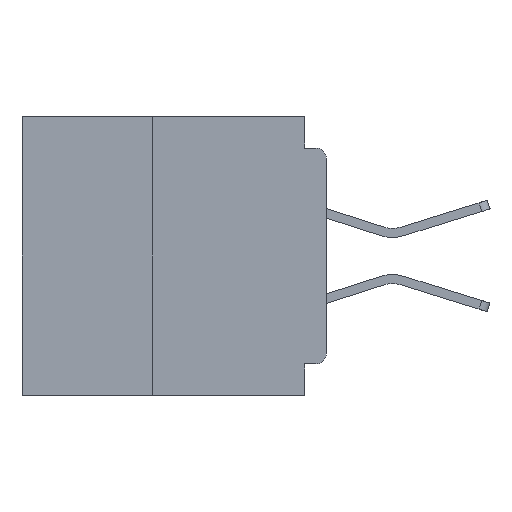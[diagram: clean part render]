
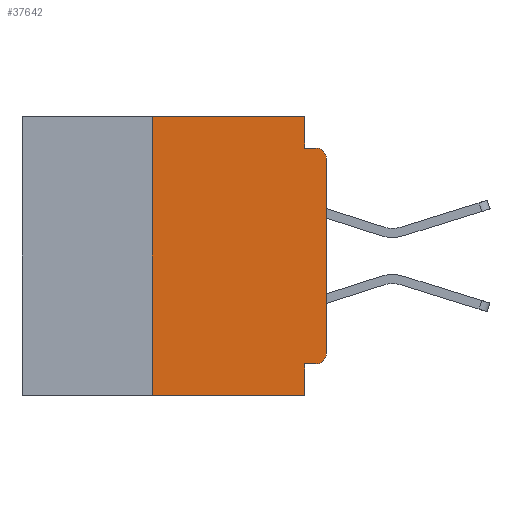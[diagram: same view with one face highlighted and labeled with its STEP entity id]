
A CAD part, left-side view. The second image highlights one B-rep face of the part: STEP entity #37642.
In plain terms, the highlighted planar face has unit normal (-1, 0, 0).
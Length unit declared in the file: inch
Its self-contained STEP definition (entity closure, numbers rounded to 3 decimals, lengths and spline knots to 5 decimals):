
#1137 = CIRCLE ( 'NONE', #14634, 0.015 ) ;
#1537 = VECTOR ( 'NONE', #10099, 39.37008 ) ;
#1831 = LINE ( 'NONE', #25739, #37626 ) ;
#2110 = ORIENTED_EDGE ( 'NONE', *, *, #35815, .F. ) ;
#2126 = EDGE_CURVE ( 'NONE', #31522, #30454, #19983, .T. ) ;
#3940 = ORIENTED_EDGE ( 'NONE', *, *, #11955, .T. ) ;
#4672 = LINE ( 'NONE', #30253, #21482 ) ;
#4858 = EDGE_CURVE ( 'NONE', #31214, #31522, #26635, .T. ) ;
#5436 = ORIENTED_EDGE ( 'NONE', *, *, #36621, .T. ) ;
#5584 = DIRECTION ( 'NONE',  ( 0., -1., 0. ) ) ;
#5889 = LINE ( 'NONE', #26978, #12720 ) ;
#6167 = LINE ( 'NONE', #42162, #40936 ) ;
#6321 = CARTESIAN_POINT ( 'NONE',  ( 0., 0.031, -0.355 ) ) ;
#6858 = ORIENTED_EDGE ( 'NONE', *, *, #15395, .F. ) ;
#7187 = CARTESIAN_POINT ( 'NONE',  ( 0., 0.015, -0.045 ) ) ;
#7306 = LINE ( 'NONE', #20938, #22028 ) ;
#7342 = DIRECTION ( 'NONE',  ( -1., 0., 0. ) ) ;
#7356 = ORIENTED_EDGE ( 'NONE', *, *, #4858, .T. ) ;
#7778 = PLANE ( 'NONE',  #36985 ) ;
#7838 = ORIENTED_EDGE ( 'NONE', *, *, #9482, .F. ) ;
#8627 = DIRECTION ( 'NONE',  ( 0., -1., 0. ) ) ;
#9482 = EDGE_CURVE ( 'NONE', #14638, #25654, #4672, .T. ) ;
#10058 = DIRECTION ( 'NONE',  ( 0., 0., -1. ) ) ;
#10099 = DIRECTION ( 'NONE',  ( 0., 1., 0. ) ) ;
#10431 = LINE ( 'NONE', #13325, #1537 ) ;
#10858 = FACE_OUTER_BOUND ( 'NONE', #35723, .T. ) ;
#11570 = VERTEX_POINT ( 'NONE', #6321 ) ;
#11955 = EDGE_CURVE ( 'NONE', #34817, #32931, #1831, .T. ) ;
#12720 = VECTOR ( 'NONE', #23538, 39.37008 ) ;
#12973 = CARTESIAN_POINT ( 'NONE',  ( 0., 0., -0.06 ) ) ;
#13325 = CARTESIAN_POINT ( 'NONE',  ( 0., 0., -0.355 ) ) ;
#14634 = AXIS2_PLACEMENT_3D ( 'NONE', #35540, #15320, #38912 ) ;
#14638 = VERTEX_POINT ( 'NONE', #20534 ) ;
#15320 = DIRECTION ( 'NONE',  ( -1., 0., 0. ) ) ;
#15395 = EDGE_CURVE ( 'NONE', #11570, #32931, #7306, .T. ) ;
#15694 = EDGE_CURVE ( 'NONE', #27826, #11570, #10431, .T. ) ;
#15885 = CARTESIAN_POINT ( 'NONE',  ( 0., 0.25, 0. ) ) ;
#17298 = ORIENTED_EDGE ( 'NONE', *, *, #32621, .F. ) ;
#17913 = DIRECTION ( 'NONE',  ( 0., 0., -1. ) ) ;
#19283 = ORIENTED_EDGE ( 'NONE', *, *, #15694, .F. ) ;
#19902 = CARTESIAN_POINT ( 'NONE',  ( 0., 0.031, -0.045 ) ) ;
#19983 = CIRCLE ( 'NONE', #32157, 0.015 ) ;
#20182 = CARTESIAN_POINT ( 'NONE',  ( 0., 0.25, -0.4 ) ) ;
#20534 = CARTESIAN_POINT ( 'NONE',  ( 0., 0.031, 0. ) ) ;
#20938 = CARTESIAN_POINT ( 'NONE',  ( 0., 0.031, -0.4 ) ) ;
#21482 = VECTOR ( 'NONE', #10058, 39.37008 ) ;
#22028 = VECTOR ( 'NONE', #34390, 39.37008 ) ;
#23538 = DIRECTION ( 'NONE',  ( 0., -1., 0. ) ) ;
#23572 = DIRECTION ( 'NONE',  ( 0., 0., 1. ) ) ;
#23615 = EDGE_CURVE ( 'NONE', #34817, #24112, #23624, .T. ) ;
#23624 = LINE ( 'NONE', #20182, #31622 ) ;
#24112 = VERTEX_POINT ( 'NONE', #15885 ) ;
#24630 = CARTESIAN_POINT ( 'NONE',  ( 0., 0., -0.34 ) ) ;
#24822 = CARTESIAN_POINT ( 'NONE',  ( 0., 0.25, -0.4 ) ) ;
#25009 = ORIENTED_EDGE ( 'NONE', *, *, #23615, .F. ) ;
#25654 = VERTEX_POINT ( 'NONE', #19902 ) ;
#25739 = CARTESIAN_POINT ( 'NONE',  ( 0., 0.437, -0.4 ) ) ;
#26635 = LINE ( 'NONE', #28516, #33485 ) ;
#26978 = CARTESIAN_POINT ( 'NONE',  ( 0., 0.437, 0. ) ) ;
#27516 = CARTESIAN_POINT ( 'NONE',  ( 0., 0.015, -0.06 ) ) ;
#27826 = VERTEX_POINT ( 'NONE', #42843 ) ;
#28182 = ORIENTED_EDGE ( 'NONE', *, *, #2126, .T. ) ;
#28516 = CARTESIAN_POINT ( 'NONE',  ( 0., 0., 0. ) ) ;
#30253 = CARTESIAN_POINT ( 'NONE',  ( 0., 0.031, 0. ) ) ;
#30454 = VERTEX_POINT ( 'NONE', #7187 ) ;
#30939 = DIRECTION ( 'NONE',  ( 0., 0., -1. ) ) ;
#31214 = VERTEX_POINT ( 'NONE', #24630 ) ;
#31218 = CARTESIAN_POINT ( 'NONE',  ( 0., 0.437, 0. ) ) ;
#31522 = VERTEX_POINT ( 'NONE', #12973 ) ;
#31622 = VECTOR ( 'NONE', #23572, 39.37008 ) ;
#32157 = AXIS2_PLACEMENT_3D ( 'NONE', #27516, #7342, #30939 ) ;
#32621 = EDGE_CURVE ( 'NONE', #25654, #30454, #6167, .T. ) ;
#32931 = VERTEX_POINT ( 'NONE', #37634 ) ;
#33485 = VECTOR ( 'NONE', #35281, 39.37008 ) ;
#34390 = DIRECTION ( 'NONE',  ( 0., 0., -1. ) ) ;
#34817 = VERTEX_POINT ( 'NONE', #24822 ) ;
#35281 = DIRECTION ( 'NONE',  ( 0., 0., 1. ) ) ;
#35540 = CARTESIAN_POINT ( 'NONE',  ( 0., 0.015, -0.34 ) ) ;
#35723 = EDGE_LOOP ( 'NONE', ( #7356, #28182, #17298, #7838, #2110, #25009, #3940, #6858, #19283, #5436 ) ) ;
#35815 = EDGE_CURVE ( 'NONE', #24112, #14638, #5889, .T. ) ;
#36621 = EDGE_CURVE ( 'NONE', #27826, #31214, #1137, .T. ) ;
#36985 = AXIS2_PLACEMENT_3D ( 'NONE', #31218, #38107, #17913 ) ;
#37626 = VECTOR ( 'NONE', #5584, 39.37008 ) ;
#37634 = CARTESIAN_POINT ( 'NONE',  ( 0., 0.031, -0.4 ) ) ;
#37642 = ADVANCED_FACE ( 'NONE', ( #10858 ), #7778, .F. ) ;
#38107 = DIRECTION ( 'NONE',  ( 1., 0., 0. ) ) ;
#38912 = DIRECTION ( 'NONE',  ( 0., 0., -1. ) ) ;
#40936 = VECTOR ( 'NONE', #8627, 39.37008 ) ;
#42162 = CARTESIAN_POINT ( 'NONE',  ( 0., 0., -0.045 ) ) ;
#42843 = CARTESIAN_POINT ( 'NONE',  ( 0., 0.015, -0.355 ) ) ;
